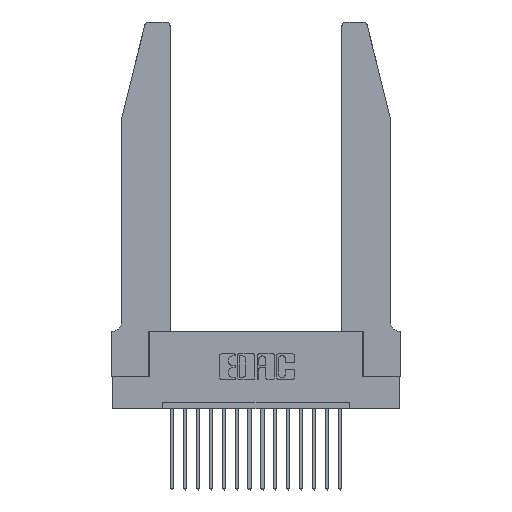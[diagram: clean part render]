
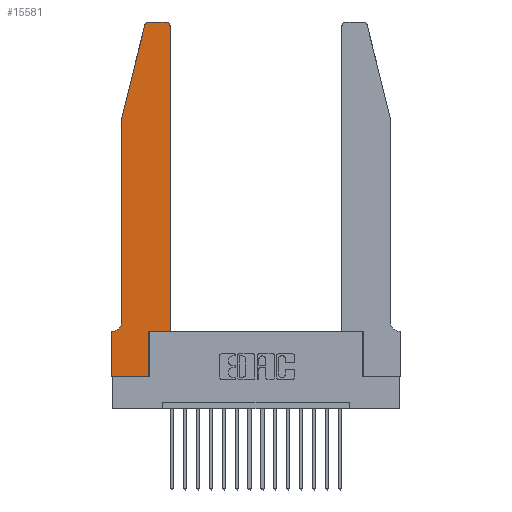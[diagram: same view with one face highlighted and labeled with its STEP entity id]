
A CAD part, top view. The second image highlights one B-rep face of the part: STEP entity #15581.
In plain terms, the highlighted planar face has unit normal (0, 0, 1).
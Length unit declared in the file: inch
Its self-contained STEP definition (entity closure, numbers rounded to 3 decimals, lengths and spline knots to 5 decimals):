
#372 = ORIENTED_EDGE ( 'NONE', *, *, #5317, .T. ) ;
#377 = VERTEX_POINT ( 'NONE', #8655 ) ;
#718 = LINE ( 'NONE', #3986, #1409 ) ;
#873 = DIRECTION ( 'NONE',  ( 1., 0., 0. ) ) ;
#1103 = CARTESIAN_POINT ( 'NONE',  ( 0., 0.35, 0.37 ) ) ;
#1141 = VECTOR ( 'NONE', #9647, 39.37008 ) ;
#1272 = VERTEX_POINT ( 'NONE', #2437 ) ;
#1311 = LINE ( 'NONE', #18536, #6998 ) ;
#1343 = DIRECTION ( 'NONE',  ( -1., 0., 0. ) ) ;
#1409 = VECTOR ( 'NONE', #5481, 39.37008 ) ;
#1772 = EDGE_CURVE ( 'NONE', #7990, #17300, #7336, .T. ) ;
#1892 = CARTESIAN_POINT ( 'NONE',  ( 0.4505, 0.35, 0.37 ) ) ;
#2346 = VECTOR ( 'NONE', #4610, 39.37008 ) ;
#2437 = CARTESIAN_POINT ( 'NONE',  ( 0.25487, 2.72718, 0.37 ) ) ;
#2569 = DIRECTION ( 'NONE',  ( 0., -1., 0. ) ) ;
#2677 = ORIENTED_EDGE ( 'NONE', *, *, #13177, .T. ) ;
#2736 = AXIS2_PLACEMENT_3D ( 'NONE', #1103, #5595, #5479 ) ;
#2823 = DIRECTION ( 'NONE',  ( 0., 0., 1. ) ) ;
#2890 = EDGE_CURVE ( 'NONE', #17300, #7606, #4046, .T. ) ;
#2975 = CARTESIAN_POINT ( 'NONE',  ( 0.0755, 0.35, 0.37 ) ) ;
#3137 = AXIS2_PLACEMENT_3D ( 'NONE', #5067, #9469, #873 ) ;
#3451 = ORIENTED_EDGE ( 'NONE', *, *, #1772, .T. ) ;
#3986 = CARTESIAN_POINT ( 'NONE',  ( 0.4505, 0.35, 0.37 ) ) ;
#4046 = LINE ( 'NONE', #2975, #4991 ) ;
#4115 = PLANE ( 'NONE',  #2736 ) ;
#4133 = CARTESIAN_POINT ( 'NONE',  ( 0.0755, 2., 0.37 ) ) ;
#4181 = EDGE_LOOP ( 'NONE', ( #4917, #12250, #10498, #372, #3451, #9055, #11911, #11780, #8567, #13516, #10673, #2677 ) ) ;
#4610 = DIRECTION ( 'NONE',  ( 0., 1., 0. ) ) ;
#4815 = CARTESIAN_POINT ( 'NONE',  ( 0.2865, 0.35, 0.37 ) ) ;
#4917 = ORIENTED_EDGE ( 'NONE', *, *, #12780, .T. ) ;
#4926 = VERTEX_POINT ( 'NONE', #14901 ) ;
#4991 = VECTOR ( 'NONE', #11992, 39.37008 ) ;
#5067 = CARTESIAN_POINT ( 'NONE',  ( 0.284, 2.72, 0.37 ) ) ;
#5317 = EDGE_CURVE ( 'NONE', #12470, #7990, #10425, .T. ) ;
#5334 = CARTESIAN_POINT ( 'NONE',  ( 0.4505, 2.72, 0.37 ) ) ;
#5457 = CARTESIAN_POINT ( 'NONE',  ( 0.0055, 0.42, 0.37 ) ) ;
#5458 = LINE ( 'NONE', #4815, #11882 ) ;
#5479 = DIRECTION ( 'NONE',  ( 1., 0., 0. ) ) ;
#5481 = DIRECTION ( 'NONE',  ( 1., 0., 0. ) ) ;
#5595 = DIRECTION ( 'NONE',  ( 0., 0., 1. ) ) ;
#5903 = VECTOR ( 'NONE', #8589, 39.37008 ) ;
#5958 = EDGE_CURVE ( 'NONE', #18757, #17909, #8279, .T. ) ;
#6354 = CIRCLE ( 'NONE', #3137, 0.03 ) ;
#6727 = CARTESIAN_POINT ( 'NONE',  ( 0.2865, 0.35, 0.37 ) ) ;
#6767 = CARTESIAN_POINT ( 'NONE',  ( 0.0755, 0.42, 0.37 ) ) ;
#6902 = CARTESIAN_POINT ( 'NONE',  ( 0.0755, 2., 0.37 ) ) ;
#6998 = VECTOR ( 'NONE', #18722, 39.37008 ) ;
#7330 = EDGE_CURVE ( 'NONE', #4926, #377, #17251, .T. ) ;
#7336 = CIRCLE ( 'NONE', #15291, 0.07 ) ;
#7449 = EDGE_CURVE ( 'NONE', #7606, #4926, #15625, .T. ) ;
#7606 = VERTEX_POINT ( 'NONE', #16339 ) ;
#7707 = DIRECTION ( 'NONE',  ( 0., 1., 0. ) ) ;
#7933 = VERTEX_POINT ( 'NONE', #17657 ) ;
#7942 = LINE ( 'NONE', #4133, #5903 ) ;
#7990 = VERTEX_POINT ( 'NONE', #6767 ) ;
#7999 = VECTOR ( 'NONE', #13549, 39.37008 ) ;
#8279 = LINE ( 'NONE', #14930, #2346 ) ;
#8567 = ORIENTED_EDGE ( 'NONE', *, *, #12975, .T. ) ;
#8589 = DIRECTION ( 'NONE',  ( -0.239, -0.971, 0. ) ) ;
#8655 = CARTESIAN_POINT ( 'NONE',  ( 0.2865, 0., 0.37 ) ) ;
#9033 = VECTOR ( 'NONE', #2569, 39.37008 ) ;
#9055 = ORIENTED_EDGE ( 'NONE', *, *, #2890, .T. ) ;
#9460 = EDGE_CURVE ( 'NONE', #12995, #18757, #718, .T. ) ;
#9469 = DIRECTION ( 'NONE',  ( 0., 0., 1. ) ) ;
#9647 = DIRECTION ( 'NONE',  ( 1., 0., 0. ) ) ;
#10425 = LINE ( 'NONE', #6902, #9033 ) ;
#10498 = ORIENTED_EDGE ( 'NONE', *, *, #12138, .T. ) ;
#10673 = ORIENTED_EDGE ( 'NONE', *, *, #5958, .T. ) ;
#10722 = CIRCLE ( 'NONE', #11693, 0.03 ) ;
#10983 = CARTESIAN_POINT ( 'NONE',  ( 0.4205, 2.72, 0.37 ) ) ;
#11577 = CARTESIAN_POINT ( 'NONE',  ( 0.284, 2.75, 0.37 ) ) ;
#11693 = AXIS2_PLACEMENT_3D ( 'NONE', #10983, #2823, #18388 ) ;
#11780 = ORIENTED_EDGE ( 'NONE', *, *, #7330, .T. ) ;
#11882 = VECTOR ( 'NONE', #7707, 39.37008 ) ;
#11911 = ORIENTED_EDGE ( 'NONE', *, *, #7449, .T. ) ;
#11992 = DIRECTION ( 'NONE',  ( -1., 0., 0. ) ) ;
#11995 = CARTESIAN_POINT ( 'NONE',  ( 0., 0., 0.37 ) ) ;
#12138 = EDGE_CURVE ( 'NONE', #1272, #12470, #7942, .T. ) ;
#12250 = ORIENTED_EDGE ( 'NONE', *, *, #16620, .T. ) ;
#12470 = VERTEX_POINT ( 'NONE', #17573 ) ;
#12780 = EDGE_CURVE ( 'NONE', #7933, #13778, #1311, .T. ) ;
#12848 = CARTESIAN_POINT ( 'NONE',  ( 0.0055, 0.35, 0.37 ) ) ;
#12975 = EDGE_CURVE ( 'NONE', #377, #12995, #5458, .T. ) ;
#12995 = VERTEX_POINT ( 'NONE', #6727 ) ;
#13177 = EDGE_CURVE ( 'NONE', #17909, #7933, #10722, .T. ) ;
#13516 = ORIENTED_EDGE ( 'NONE', *, *, #9460, .T. ) ;
#13549 = DIRECTION ( 'NONE',  ( 0., -1., 0. ) ) ;
#13778 = VERTEX_POINT ( 'NONE', #11577 ) ;
#14901 = CARTESIAN_POINT ( 'NONE',  ( 0., 0., 0.37 ) ) ;
#14930 = CARTESIAN_POINT ( 'NONE',  ( 0.4505, 0.35, 0.37 ) ) ;
#15291 = AXIS2_PLACEMENT_3D ( 'NONE', #5457, #17416, #1343 ) ;
#15581 = ADVANCED_FACE ( 'NONE', ( #17999 ), #4115, .T. ) ;
#15625 = LINE ( 'NONE', #11995, #7999 ) ;
#16339 = CARTESIAN_POINT ( 'NONE',  ( 0., 0.35, 0.37 ) ) ;
#16620 = EDGE_CURVE ( 'NONE', #13778, #1272, #6354, .T. ) ;
#17251 = LINE ( 'NONE', #18351, #1141 ) ;
#17300 = VERTEX_POINT ( 'NONE', #12848 ) ;
#17416 = DIRECTION ( 'NONE',  ( 0., 0., -1. ) ) ;
#17573 = CARTESIAN_POINT ( 'NONE',  ( 0.0755, 2., 0.37 ) ) ;
#17657 = CARTESIAN_POINT ( 'NONE',  ( 0.4205, 2.75, 0.37 ) ) ;
#17909 = VERTEX_POINT ( 'NONE', #5334 ) ;
#17999 = FACE_OUTER_BOUND ( 'NONE', #4181, .T. ) ;
#18351 = CARTESIAN_POINT ( 'NONE',  ( 0., 0., 0.37 ) ) ;
#18388 = DIRECTION ( 'NONE',  ( 1., 0., 0. ) ) ;
#18536 = CARTESIAN_POINT ( 'NONE',  ( 0.2605, 2.75, 0.37 ) ) ;
#18722 = DIRECTION ( 'NONE',  ( -1., 0., 0. ) ) ;
#18757 = VERTEX_POINT ( 'NONE', #1892 ) ;
